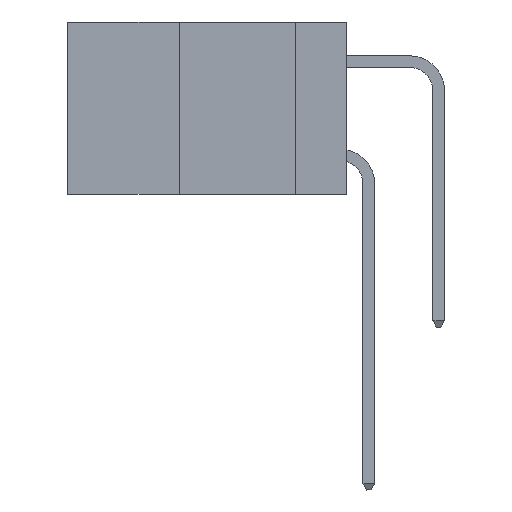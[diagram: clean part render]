
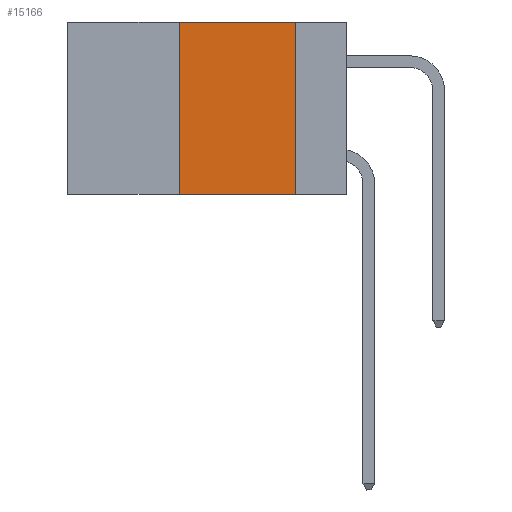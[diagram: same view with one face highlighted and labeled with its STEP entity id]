
A CAD part, left-side view. The second image highlights one B-rep face of the part: STEP entity #15166.
In plain terms, the highlighted planar face has unit normal (-1, 0, 0).
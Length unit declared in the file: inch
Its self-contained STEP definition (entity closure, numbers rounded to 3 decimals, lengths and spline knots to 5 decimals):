
#688 = CARTESIAN_POINT ( 'NONE',  ( 0., 0.11, 0. ) ) ;
#912 = ORIENTED_EDGE ( 'NONE', *, *, #23595, .F. ) ;
#1397 = CARTESIAN_POINT ( 'NONE',  ( 0., 0.6, 0. ) ) ;
#1562 = ORIENTED_EDGE ( 'NONE', *, *, #4502, .F. ) ;
#1789 = CARTESIAN_POINT ( 'NONE',  ( 0., 0.11, -0.37 ) ) ;
#2092 = EDGE_LOOP ( 'NONE', ( #4747, #912, #1562, #6409 ) ) ;
#2430 = LINE ( 'NONE', #21745, #10536 ) ;
#2917 = LINE ( 'NONE', #1397, #3048 ) ;
#3048 = VECTOR ( 'NONE', #6691, 39.37008 ) ;
#3221 = VERTEX_POINT ( 'NONE', #688 ) ;
#4502 = EDGE_CURVE ( 'NONE', #21141, #23822, #2430, .T. ) ;
#4747 = ORIENTED_EDGE ( 'NONE', *, *, #19109, .F. ) ;
#5993 = CARTESIAN_POINT ( 'NONE',  ( 0., 0.6, -0.37 ) ) ;
#6409 = ORIENTED_EDGE ( 'NONE', *, *, #8455, .T. ) ;
#6691 = DIRECTION ( 'NONE',  ( 0., -1., 0. ) ) ;
#6820 = DIRECTION ( 'NONE',  ( 0., 0., -1. ) ) ;
#8455 = EDGE_CURVE ( 'NONE', #21141, #21912, #23158, .T. ) ;
#10073 = DIRECTION ( 'NONE',  ( 1., 0., 0. ) ) ;
#10536 = VECTOR ( 'NONE', #17745, 39.37008 ) ;
#11915 = AXIS2_PLACEMENT_3D ( 'NONE', #17707, #10073, #23479 ) ;
#13632 = DIRECTION ( 'NONE',  ( 0., -1., 0. ) ) ;
#15017 = CARTESIAN_POINT ( 'NONE',  ( 0., 0.36, -0.37 ) ) ;
#15166 = ADVANCED_FACE ( 'NONE', ( #23350 ), #15828, .F. ) ;
#15666 = VECTOR ( 'NONE', #13632, 39.37008 ) ;
#15828 = PLANE ( 'NONE',  #11915 ) ;
#16225 = LINE ( 'NONE', #23995, #19373 ) ;
#17707 = CARTESIAN_POINT ( 'NONE',  ( 0., 0.6, 0. ) ) ;
#17745 = DIRECTION ( 'NONE',  ( 0., 0., 1. ) ) ;
#19109 = EDGE_CURVE ( 'NONE', #3221, #21912, #16225, .T. ) ;
#19373 = VECTOR ( 'NONE', #6820, 39.37008 ) ;
#21141 = VERTEX_POINT ( 'NONE', #15017 ) ;
#21319 = CARTESIAN_POINT ( 'NONE',  ( 0., 0.36, 0. ) ) ;
#21745 = CARTESIAN_POINT ( 'NONE',  ( 0., 0.36, 0. ) ) ;
#21912 = VERTEX_POINT ( 'NONE', #1789 ) ;
#23158 = LINE ( 'NONE', #5993, #15666 ) ;
#23350 = FACE_OUTER_BOUND ( 'NONE', #2092, .T. ) ;
#23479 = DIRECTION ( 'NONE',  ( 0., 0., -1. ) ) ;
#23595 = EDGE_CURVE ( 'NONE', #23822, #3221, #2917, .T. ) ;
#23822 = VERTEX_POINT ( 'NONE', #21319 ) ;
#23995 = CARTESIAN_POINT ( 'NONE',  ( 0., 0.11, 0. ) ) ;
